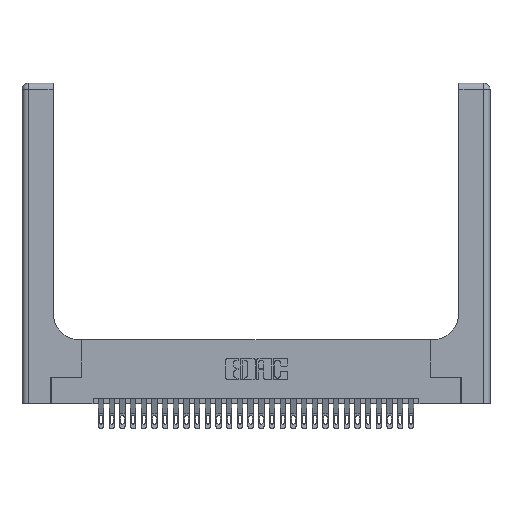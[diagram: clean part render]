
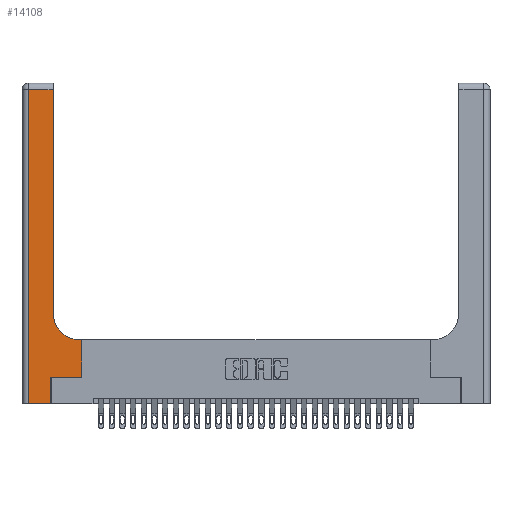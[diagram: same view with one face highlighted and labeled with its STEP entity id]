
A CAD part, top view. The second image highlights one B-rep face of the part: STEP entity #14108.
In plain terms, the highlighted planar face has unit normal (0, 0, 1).
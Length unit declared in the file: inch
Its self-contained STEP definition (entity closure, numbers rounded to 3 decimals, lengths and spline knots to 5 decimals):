
#225 = CARTESIAN_POINT ( 'NONE',  ( 0.5415, 0.85, 0.37 ) ) ;
#428 = DIRECTION ( 'NONE',  ( -1., 0., 0. ) ) ;
#801 = PLANE ( 'NONE',  #17931 ) ;
#813 = CARTESIAN_POINT ( 'NONE',  ( 0.06, 3., 0.37 ) ) ;
#858 = LINE ( 'NONE', #21733, #28660 ) ;
#1009 = DIRECTION ( 'NONE',  ( 0., -1., 0. ) ) ;
#1112 = VERTEX_POINT ( 'NONE', #1298 ) ;
#1298 = CARTESIAN_POINT ( 'NONE',  ( 0.5585, 0.25, 0.37 ) ) ;
#1480 = ORIENTED_EDGE ( 'NONE', *, *, #27147, .T. ) ;
#2167 = EDGE_CURVE ( 'NONE', #1112, #20550, #28803, .T. ) ;
#3311 = CARTESIAN_POINT ( 'NONE',  ( 0., 0., 0.37 ) ) ;
#3377 = DIRECTION ( 'NONE',  ( 0., 1., 0. ) ) ;
#3606 = ORIENTED_EDGE ( 'NONE', *, *, #21924, .T. ) ;
#4008 = VECTOR ( 'NONE', #20759, 39.37008 ) ;
#5355 = ORIENTED_EDGE ( 'NONE', *, *, #10996, .T. ) ;
#5469 = CIRCLE ( 'NONE', #12778, 0.25 ) ;
#5890 = ORIENTED_EDGE ( 'NONE', *, *, #9252, .T. ) ;
#6016 = DIRECTION ( 'NONE',  ( -1., 0., 0. ) ) ;
#6639 = EDGE_CURVE ( 'NONE', #20550, #19003, #8600, .T. ) ;
#6709 = VECTOR ( 'NONE', #1009, 39.37008 ) ;
#7288 = VECTOR ( 'NONE', #30452, 39.37008 ) ;
#7300 = CARTESIAN_POINT ( 'NONE',  ( 0.2915, 0.6, 0.37 ) ) ;
#7597 = CARTESIAN_POINT ( 'NONE',  ( 0.2915, 3., 0.37 ) ) ;
#8424 = VERTEX_POINT ( 'NONE', #18559 ) ;
#8600 = LINE ( 'NONE', #7300, #29346 ) ;
#9252 = EDGE_CURVE ( 'NONE', #15844, #13167, #14665, .T. ) ;
#9390 = EDGE_CURVE ( 'NONE', #14150, #21150, #26896, .T. ) ;
#9798 = DIRECTION ( 'NONE',  ( 1., 0., 0. ) ) ;
#10307 = LINE ( 'NONE', #13784, #4008 ) ;
#10338 = CARTESIAN_POINT ( 'NONE',  ( 0.269, 0., 0.37 ) ) ;
#10996 = EDGE_CURVE ( 'NONE', #13167, #24668, #858, .T. ) ;
#11293 = ORIENTED_EDGE ( 'NONE', *, *, #26429, .T. ) ;
#11355 = EDGE_CURVE ( 'NONE', #24668, #8424, #27508, .T. ) ;
#11509 = ORIENTED_EDGE ( 'NONE', *, *, #2167, .T. ) ;
#12778 = AXIS2_PLACEMENT_3D ( 'NONE', #225, #16871, #9798 ) ;
#13091 = CARTESIAN_POINT ( 'NONE',  ( 0.5415, 0.6, 0.37 ) ) ;
#13167 = VERTEX_POINT ( 'NONE', #14823 ) ;
#13784 = CARTESIAN_POINT ( 'NONE',  ( 0.269, 0.25, 0.37 ) ) ;
#14108 = ADVANCED_FACE ( 'NONE', ( #26285 ), #801, .F. ) ;
#14150 = VERTEX_POINT ( 'NONE', #10338 ) ;
#14217 = CARTESIAN_POINT ( 'NONE',  ( 0.2915, 0.85, 0.37 ) ) ;
#14665 = LINE ( 'NONE', #7597, #28785 ) ;
#14823 = CARTESIAN_POINT ( 'NONE',  ( 0.2915, 2.94, 0.37 ) ) ;
#15844 = VERTEX_POINT ( 'NONE', #14217 ) ;
#16871 = DIRECTION ( 'NONE',  ( 0., 0., -1. ) ) ;
#17497 = VECTOR ( 'NONE', #24703, 39.37008 ) ;
#17931 = AXIS2_PLACEMENT_3D ( 'NONE', #29094, #21964, #29287 ) ;
#18559 = CARTESIAN_POINT ( 'NONE',  ( 0.06, 0., 0.37 ) ) ;
#18793 = CARTESIAN_POINT ( 'NONE',  ( 0.5585, 0.25, 0.37 ) ) ;
#19003 = VERTEX_POINT ( 'NONE', #13091 ) ;
#20550 = VERTEX_POINT ( 'NONE', #23042 ) ;
#20759 = DIRECTION ( 'NONE',  ( 1., 0., 0. ) ) ;
#21150 = VERTEX_POINT ( 'NONE', #23020 ) ;
#21726 = ORIENTED_EDGE ( 'NONE', *, *, #6639, .T. ) ;
#21733 = CARTESIAN_POINT ( 'NONE',  ( 0., 2.94, 0.37 ) ) ;
#21924 = EDGE_CURVE ( 'NONE', #8424, #14150, #23067, .T. ) ;
#21964 = DIRECTION ( 'NONE',  ( 0., 0., -1. ) ) ;
#23020 = CARTESIAN_POINT ( 'NONE',  ( 0.269, 0.25, 0.37 ) ) ;
#23042 = CARTESIAN_POINT ( 'NONE',  ( 0.5585, 0.6, 0.37 ) ) ;
#23067 = LINE ( 'NONE', #3311, #17497 ) ;
#24668 = VERTEX_POINT ( 'NONE', #27504 ) ;
#24703 = DIRECTION ( 'NONE',  ( 1., 0., 0. ) ) ;
#25001 = ORIENTED_EDGE ( 'NONE', *, *, #11355, .T. ) ;
#26285 = FACE_OUTER_BOUND ( 'NONE', #29074, .T. ) ;
#26429 = EDGE_CURVE ( 'NONE', #21150, #1112, #10307, .T. ) ;
#26634 = CARTESIAN_POINT ( 'NONE',  ( 0.269, 0., 0.37 ) ) ;
#26735 = DIRECTION ( 'NONE',  ( 0., 1., 0. ) ) ;
#26896 = LINE ( 'NONE', #26634, #27624 ) ;
#27147 = EDGE_CURVE ( 'NONE', #19003, #15844, #5469, .T. ) ;
#27504 = CARTESIAN_POINT ( 'NONE',  ( 0.06, 2.94, 0.37 ) ) ;
#27508 = LINE ( 'NONE', #813, #6709 ) ;
#27624 = VECTOR ( 'NONE', #26735, 39.37008 ) ;
#28660 = VECTOR ( 'NONE', #428, 39.37008 ) ;
#28785 = VECTOR ( 'NONE', #3377, 39.37008 ) ;
#28803 = LINE ( 'NONE', #18793, #7288 ) ;
#29074 = EDGE_LOOP ( 'NONE', ( #5890, #5355, #25001, #3606, #29093, #11293, #11509, #21726, #1480 ) ) ;
#29093 = ORIENTED_EDGE ( 'NONE', *, *, #9390, .T. ) ;
#29094 = CARTESIAN_POINT ( 'NONE',  ( 0., 3., 0.37 ) ) ;
#29287 = DIRECTION ( 'NONE',  ( -1., 0., 0. ) ) ;
#29346 = VECTOR ( 'NONE', #6016, 39.37008 ) ;
#30452 = DIRECTION ( 'NONE',  ( 0., 1., 0. ) ) ;
